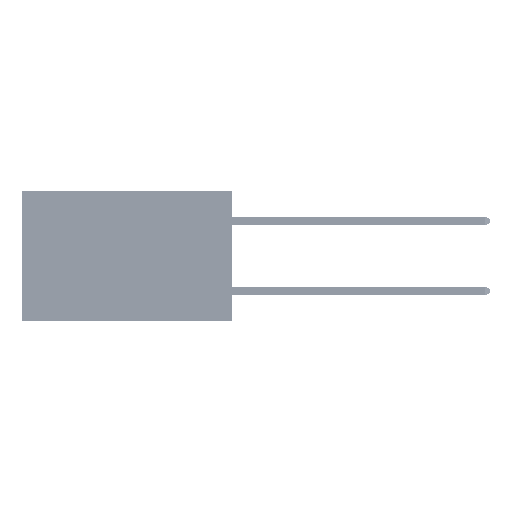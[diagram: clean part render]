
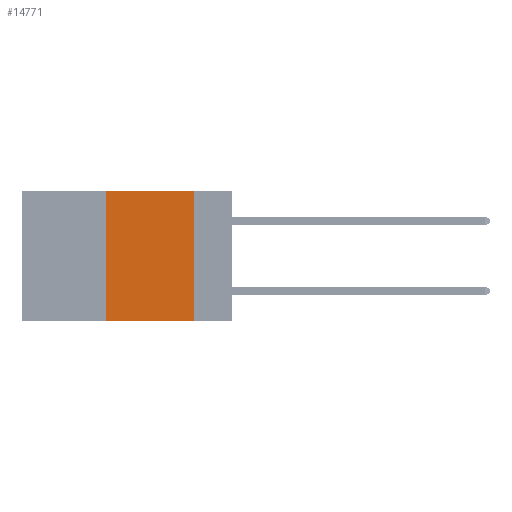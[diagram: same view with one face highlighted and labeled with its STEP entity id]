
A CAD part, left-side view. The second image highlights one B-rep face of the part: STEP entity #14771.
In plain terms, the highlighted planar face has unit normal (-1, 0, 0).
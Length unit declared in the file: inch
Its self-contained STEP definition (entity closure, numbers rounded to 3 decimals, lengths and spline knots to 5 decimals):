
#2368 = EDGE_CURVE ( 'NONE', #32411, #45234, #49756, .T. ) ;
#7114 = CARTESIAN_POINT ( 'NONE',  ( 0., 0.11, 0. ) ) ;
#9635 = VECTOR ( 'NONE', #20742, 39.37008 ) ;
#12009 = VERTEX_POINT ( 'NONE', #41849 ) ;
#14675 = VERTEX_POINT ( 'NONE', #40589 ) ;
#14771 = ADVANCED_FACE ( 'NONE', ( #18500 ), #37637, .F. ) ;
#15290 = LINE ( 'NONE', #29003, #41664 ) ;
#16664 = CARTESIAN_POINT ( 'NONE',  ( 0., 0.36, 0. ) ) ;
#17441 = CARTESIAN_POINT ( 'NONE',  ( 0., 0.6, 0. ) ) ;
#18500 = FACE_OUTER_BOUND ( 'NONE', #48804, .T. ) ;
#20681 = EDGE_CURVE ( 'NONE', #45234, #12009, #38776, .T. ) ;
#20742 = DIRECTION ( 'NONE',  ( 0., -1., 0. ) ) ;
#22125 = LINE ( 'NONE', #32545, #9635 ) ;
#22624 = CARTESIAN_POINT ( 'NONE',  ( 0., 0.6, 0. ) ) ;
#23448 = EDGE_CURVE ( 'NONE', #14675, #32411, #15290, .T. ) ;
#24351 = ORIENTED_EDGE ( 'NONE', *, *, #20681, .F. ) ;
#26337 = CARTESIAN_POINT ( 'NONE',  ( 0., 0.11, 0. ) ) ;
#26851 = DIRECTION ( 'NONE',  ( 0., -1., 0. ) ) ;
#29003 = CARTESIAN_POINT ( 'NONE',  ( 0., 0.36, 0. ) ) ;
#32411 = VERTEX_POINT ( 'NONE', #16664 ) ;
#32545 = CARTESIAN_POINT ( 'NONE',  ( 0., 0.6, -0.37 ) ) ;
#32658 = ORIENTED_EDGE ( 'NONE', *, *, #39545, .T. ) ;
#33795 = DIRECTION ( 'NONE',  ( 1., 0., 0. ) ) ;
#35522 = DIRECTION ( 'NONE',  ( 0., 0., -1. ) ) ;
#37637 = PLANE ( 'NONE',  #51729 ) ;
#38776 = LINE ( 'NONE', #7114, #40003 ) ;
#39545 = EDGE_CURVE ( 'NONE', #14675, #12009, #22125, .T. ) ;
#40003 = VECTOR ( 'NONE', #35522, 39.37008 ) ;
#40589 = CARTESIAN_POINT ( 'NONE',  ( 0., 0.36, -0.37 ) ) ;
#41470 = DIRECTION ( 'NONE',  ( 0., 0., 1. ) ) ;
#41588 = ORIENTED_EDGE ( 'NONE', *, *, #2368, .F. ) ;
#41664 = VECTOR ( 'NONE', #41470, 39.37008 ) ;
#41849 = CARTESIAN_POINT ( 'NONE',  ( 0., 0.11, -0.37 ) ) ;
#43112 = ORIENTED_EDGE ( 'NONE', *, *, #23448, .F. ) ;
#45234 = VERTEX_POINT ( 'NONE', #26337 ) ;
#47841 = VECTOR ( 'NONE', #26851, 39.37008 ) ;
#48804 = EDGE_LOOP ( 'NONE', ( #24351, #41588, #43112, #32658 ) ) ;
#49756 = LINE ( 'NONE', #22624, #47841 ) ;
#50273 = DIRECTION ( 'NONE',  ( 0., 0., -1. ) ) ;
#51729 = AXIS2_PLACEMENT_3D ( 'NONE', #17441, #33795, #50273 ) ;
